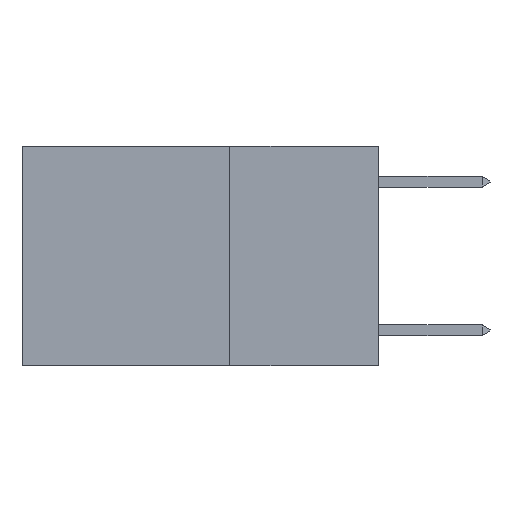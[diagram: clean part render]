
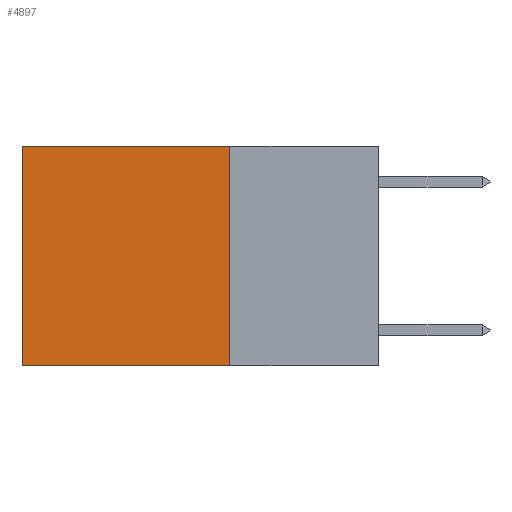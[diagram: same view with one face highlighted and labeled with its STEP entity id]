
A CAD part, left-side view. The second image highlights one B-rep face of the part: STEP entity #4897.
In plain terms, the highlighted planar face has unit normal (-1, 0, 0).
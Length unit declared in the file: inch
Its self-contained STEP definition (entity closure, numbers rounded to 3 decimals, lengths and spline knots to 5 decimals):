
#554 = FACE_OUTER_BOUND ( 'NONE', #9585, .T. ) ;
#3774 = CARTESIAN_POINT ( 'NONE',  ( 0.2625, 0.25, 0. ) ) ;
#4897 = ADVANCED_FACE ( 'NONE', ( #554 ), #28182, .F. ) ;
#6257 = EDGE_CURVE ( 'NONE', #13635, #18686, #15533, .T. ) ;
#6866 = VERTEX_POINT ( 'NONE', #9687 ) ;
#7283 = VECTOR ( 'NONE', #21103, 39.37008 ) ;
#8915 = DIRECTION ( 'NONE',  ( 0., 0., -1. ) ) ;
#9257 = ORIENTED_EDGE ( 'NONE', *, *, #12998, .T. ) ;
#9408 = VECTOR ( 'NONE', #27894, 39.37008 ) ;
#9585 = EDGE_LOOP ( 'NONE', ( #18133, #30282, #21649, #9257 ) ) ;
#9687 = CARTESIAN_POINT ( 'NONE',  ( 0.2625, 0.6, 0. ) ) ;
#11614 = LINE ( 'NONE', #28450, #16113 ) ;
#11708 = EDGE_CURVE ( 'NONE', #18482, #13635, #26796, .T. ) ;
#12394 = CARTESIAN_POINT ( 'NONE',  ( 0.2625, 0.25, -0.37 ) ) ;
#12998 = EDGE_CURVE ( 'NONE', #18482, #6866, #11614, .T. ) ;
#13301 = DIRECTION ( 'NONE',  ( 1., 0., 0. ) ) ;
#13635 = VERTEX_POINT ( 'NONE', #12394 ) ;
#15533 = LINE ( 'NONE', #29847, #7283 ) ;
#16113 = VECTOR ( 'NONE', #28340, 39.37008 ) ;
#16334 = AXIS2_PLACEMENT_3D ( 'NONE', #3774, #13301, #8915 ) ;
#16591 = VECTOR ( 'NONE', #25433, 39.37008 ) ;
#18133 = ORIENTED_EDGE ( 'NONE', *, *, #29879, .T. ) ;
#18482 = VERTEX_POINT ( 'NONE', #30061 ) ;
#18686 = VERTEX_POINT ( 'NONE', #30505 ) ;
#20630 = CARTESIAN_POINT ( 'NONE',  ( 0.2625, 0.6, 0. ) ) ;
#21103 = DIRECTION ( 'NONE',  ( 0., 1., 0. ) ) ;
#21649 = ORIENTED_EDGE ( 'NONE', *, *, #11708, .F. ) ;
#22993 = CARTESIAN_POINT ( 'NONE',  ( 0.2625, 0.25, 0. ) ) ;
#25433 = DIRECTION ( 'NONE',  ( 0., 0., -1. ) ) ;
#26796 = LINE ( 'NONE', #22993, #16591 ) ;
#27894 = DIRECTION ( 'NONE',  ( 0., 0., -1. ) ) ;
#28182 = PLANE ( 'NONE',  #16334 ) ;
#28340 = DIRECTION ( 'NONE',  ( 0., 1., 0. ) ) ;
#28450 = CARTESIAN_POINT ( 'NONE',  ( 0.2625, 0.25, 0. ) ) ;
#28649 = LINE ( 'NONE', #20630, #9408 ) ;
#29847 = CARTESIAN_POINT ( 'NONE',  ( 0.2625, 0.25, -0.37 ) ) ;
#29879 = EDGE_CURVE ( 'NONE', #6866, #18686, #28649, .T. ) ;
#30061 = CARTESIAN_POINT ( 'NONE',  ( 0.2625, 0.25, 0. ) ) ;
#30282 = ORIENTED_EDGE ( 'NONE', *, *, #6257, .F. ) ;
#30505 = CARTESIAN_POINT ( 'NONE',  ( 0.2625, 0.6, -0.37 ) ) ;
